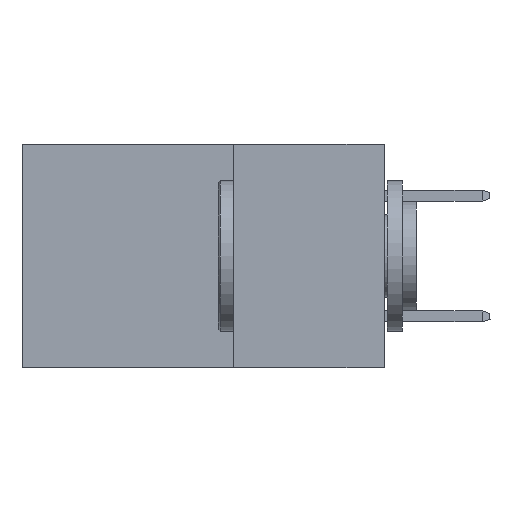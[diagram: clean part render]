
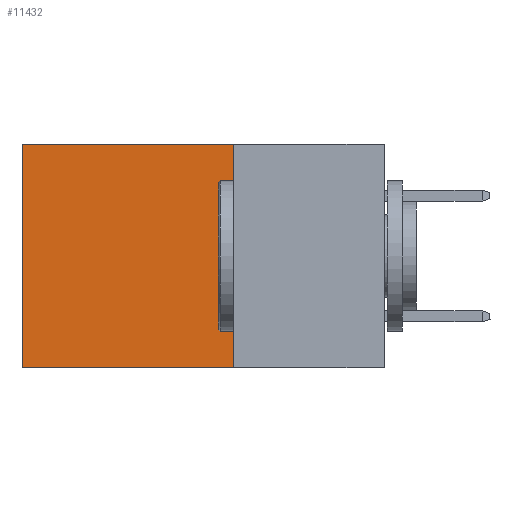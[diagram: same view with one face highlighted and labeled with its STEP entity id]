
A CAD part, left-side view. The second image highlights one B-rep face of the part: STEP entity #11432.
In plain terms, the highlighted planar face has unit normal (-1, 0, 0).
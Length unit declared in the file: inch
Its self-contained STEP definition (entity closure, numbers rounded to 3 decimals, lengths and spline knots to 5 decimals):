
#44 = DIRECTION ( 'NONE',  ( 0., 1., 0. ) ) ;
#141 = CARTESIAN_POINT ( 'NONE',  ( 0.2615, 0.25, 0. ) ) ;
#187 = CARTESIAN_POINT ( 'NONE',  ( 0.2615, 0.25, 0. ) ) ;
#653 = CARTESIAN_POINT ( 'NONE',  ( 0.2615, 0.6, 0. ) ) ;
#2069 = CARTESIAN_POINT ( 'NONE',  ( 0.2615, 0.25, -0.37 ) ) ;
#2268 = VERTEX_POINT ( 'NONE', #17807 ) ;
#3250 = EDGE_CURVE ( 'NONE', #18186, #14629, #9562, .T. ) ;
#3622 = DIRECTION ( 'NONE',  ( 0., 0., -1. ) ) ;
#3797 = EDGE_CURVE ( 'NONE', #2268, #13594, #16291, .T. ) ;
#4569 = CARTESIAN_POINT ( 'NONE',  ( 0.2615, 0.6, -0.37 ) ) ;
#5608 = VECTOR ( 'NONE', #44, 39.37008 ) ;
#6143 = EDGE_LOOP ( 'NONE', ( #10801, #6464, #10134, #7241 ) ) ;
#6432 = DIRECTION ( 'NONE',  ( 0., 0., -1. ) ) ;
#6464 = ORIENTED_EDGE ( 'NONE', *, *, #3797, .F. ) ;
#6515 = PLANE ( 'NONE',  #11618 ) ;
#7241 = ORIENTED_EDGE ( 'NONE', *, *, #3250, .T. ) ;
#7581 = CARTESIAN_POINT ( 'NONE',  ( 0.2615, 0.6, -0.37 ) ) ;
#7717 = DIRECTION ( 'NONE',  ( 0., 0., -1. ) ) ;
#9229 = EDGE_CURVE ( 'NONE', #14629, #13594, #16748, .T. ) ;
#9319 = LINE ( 'NONE', #10754, #16062 ) ;
#9562 = LINE ( 'NONE', #187, #5608 ) ;
#9926 = CARTESIAN_POINT ( 'NONE',  ( 0.2615, 0.25, -0.37 ) ) ;
#10134 = ORIENTED_EDGE ( 'NONE', *, *, #15450, .F. ) ;
#10754 = CARTESIAN_POINT ( 'NONE',  ( 0.2615, 0.25, -0.37 ) ) ;
#10801 = ORIENTED_EDGE ( 'NONE', *, *, #9229, .T. ) ;
#11432 = ADVANCED_FACE ( 'NONE', ( #13546 ), #6515, .F. ) ;
#11618 = AXIS2_PLACEMENT_3D ( 'NONE', #2069, #12356, #3622 ) ;
#12356 = DIRECTION ( 'NONE',  ( 1., 0., 0. ) ) ;
#12441 = VECTOR ( 'NONE', #16909, 39.37008 ) ;
#13546 = FACE_OUTER_BOUND ( 'NONE', #6143, .T. ) ;
#13594 = VERTEX_POINT ( 'NONE', #4569 ) ;
#14629 = VERTEX_POINT ( 'NONE', #653 ) ;
#15450 = EDGE_CURVE ( 'NONE', #18186, #2268, #9319, .T. ) ;
#16062 = VECTOR ( 'NONE', #6432, 39.37008 ) ;
#16291 = LINE ( 'NONE', #9926, #12441 ) ;
#16306 = VECTOR ( 'NONE', #7717, 39.37008 ) ;
#16748 = LINE ( 'NONE', #7581, #16306 ) ;
#16909 = DIRECTION ( 'NONE',  ( 0., 1., 0. ) ) ;
#17807 = CARTESIAN_POINT ( 'NONE',  ( 0.2615, 0.25, -0.37 ) ) ;
#18186 = VERTEX_POINT ( 'NONE', #141 ) ;
